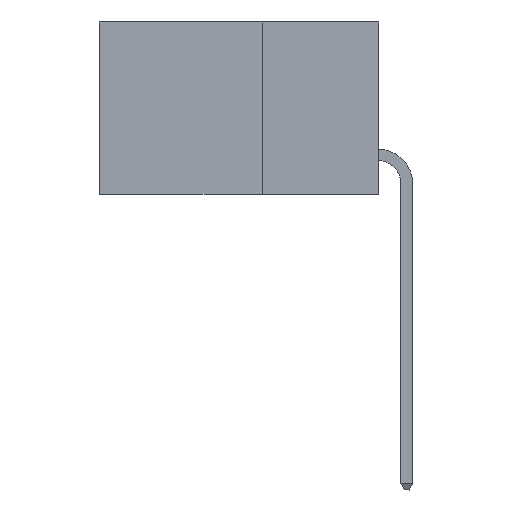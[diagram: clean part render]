
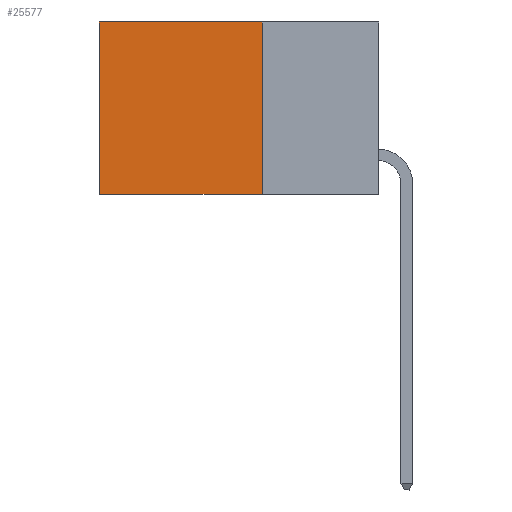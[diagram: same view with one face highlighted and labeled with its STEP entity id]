
A CAD part, left-side view. The second image highlights one B-rep face of the part: STEP entity #25577.
In plain terms, the highlighted planar face has unit normal (-1, 0, 0).
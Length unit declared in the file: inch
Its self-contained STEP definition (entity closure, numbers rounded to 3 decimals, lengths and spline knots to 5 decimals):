
#63 = ORIENTED_EDGE ( 'NONE', *, *, #12453, .T. ) ;
#803 = LINE ( 'NONE', #11853, #6889 ) ;
#1671 = DIRECTION ( 'NONE',  ( 0., 0., -1. ) ) ;
#3054 = CARTESIAN_POINT ( 'NONE',  ( 0.298, 0.25, 0. ) ) ;
#3792 = CARTESIAN_POINT ( 'NONE',  ( 0.298, 0.25, -0.37 ) ) ;
#4029 = VERTEX_POINT ( 'NONE', #8056 ) ;
#5662 = DIRECTION ( 'NONE',  ( 0., 0., -1. ) ) ;
#5837 = LINE ( 'NONE', #6720, #30796 ) ;
#6387 = DIRECTION ( 'NONE',  ( 0., 1., 0. ) ) ;
#6720 = CARTESIAN_POINT ( 'NONE',  ( 0.298, 0.25, 0. ) ) ;
#6889 = VECTOR ( 'NONE', #1671, 39.37008 ) ;
#7184 = FACE_OUTER_BOUND ( 'NONE', #29636, .T. ) ;
#7365 = EDGE_CURVE ( 'NONE', #14046, #9528, #18233, .T. ) ;
#8056 = CARTESIAN_POINT ( 'NONE',  ( 0.298, 0.6, 0. ) ) ;
#8519 = EDGE_CURVE ( 'NONE', #9528, #28933, #14689, .T. ) ;
#9528 = VERTEX_POINT ( 'NONE', #20080 ) ;
#9634 = CARTESIAN_POINT ( 'NONE',  ( 0.298, 0.6, -0.37 ) ) ;
#11853 = CARTESIAN_POINT ( 'NONE',  ( 0.298, 0.6, 0. ) ) ;
#12453 = EDGE_CURVE ( 'NONE', #14046, #4029, #5837, .T. ) ;
#13054 = PLANE ( 'NONE',  #23928 ) ;
#14046 = VERTEX_POINT ( 'NONE', #24023 ) ;
#14689 = LINE ( 'NONE', #3792, #27126 ) ;
#17170 = DIRECTION ( 'NONE',  ( 0., 0., -1. ) ) ;
#17468 = VECTOR ( 'NONE', #17170, 39.37008 ) ;
#18233 = LINE ( 'NONE', #22083, #17468 ) ;
#20080 = CARTESIAN_POINT ( 'NONE',  ( 0.298, 0.25, -0.37 ) ) ;
#20639 = DIRECTION ( 'NONE',  ( 1., 0., 0. ) ) ;
#22083 = CARTESIAN_POINT ( 'NONE',  ( 0.298, 0.25, 0. ) ) ;
#22251 = ORIENTED_EDGE ( 'NONE', *, *, #8519, .F. ) ;
#23928 = AXIS2_PLACEMENT_3D ( 'NONE', #3054, #20639, #5662 ) ;
#24023 = CARTESIAN_POINT ( 'NONE',  ( 0.298, 0.25, 0. ) ) ;
#24132 = ORIENTED_EDGE ( 'NONE', *, *, #7365, .F. ) ;
#25577 = ADVANCED_FACE ( 'NONE', ( #7184 ), #13054, .F. ) ;
#27126 = VECTOR ( 'NONE', #6387, 39.37008 ) ;
#28402 = EDGE_CURVE ( 'NONE', #4029, #28933, #803, .T. ) ;
#28933 = VERTEX_POINT ( 'NONE', #9634 ) ;
#29636 = EDGE_LOOP ( 'NONE', ( #32000, #22251, #24132, #63 ) ) ;
#30796 = VECTOR ( 'NONE', #31636, 39.37008 ) ;
#31636 = DIRECTION ( 'NONE',  ( 0., 1., 0. ) ) ;
#32000 = ORIENTED_EDGE ( 'NONE', *, *, #28402, .T. ) ;
